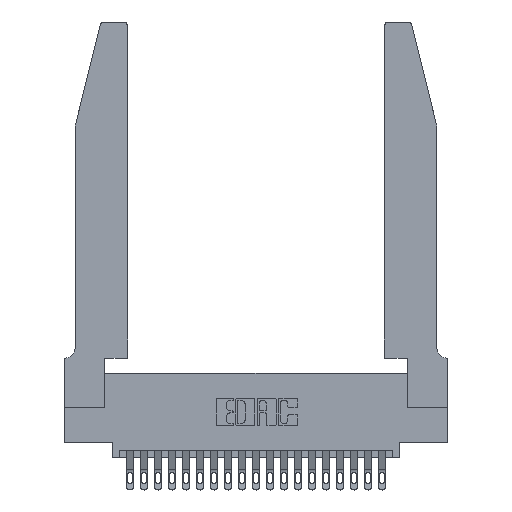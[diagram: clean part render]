
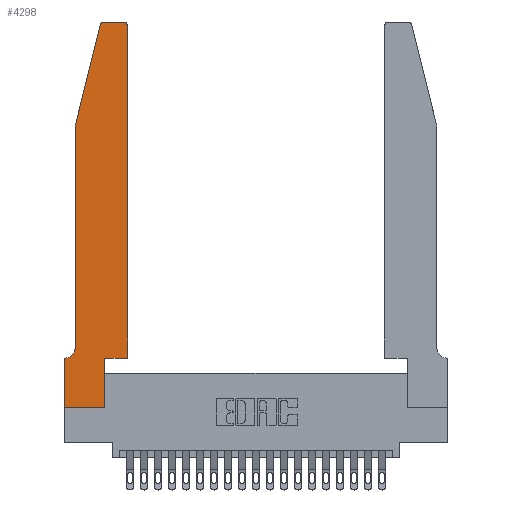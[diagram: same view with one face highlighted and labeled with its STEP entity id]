
A CAD part, top view. The second image highlights one B-rep face of the part: STEP entity #4298.
In plain terms, the highlighted planar face has unit normal (0, 0, 1).
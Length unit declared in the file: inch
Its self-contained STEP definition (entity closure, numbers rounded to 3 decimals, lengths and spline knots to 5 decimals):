
#197 = CARTESIAN_POINT ( 'NONE',  ( 0.4505, 0.35, 0.37 ) ) ;
#592 = LINE ( 'NONE', #1288, #1196 ) ;
#927 = ORIENTED_EDGE ( 'NONE', *, *, #7101, .T. ) ;
#1135 = CARTESIAN_POINT ( 'NONE',  ( 0.284, 2.72, 0.37 ) ) ;
#1196 = VECTOR ( 'NONE', #13981, 39.37008 ) ;
#1288 = CARTESIAN_POINT ( 'NONE',  ( 0., 0., 0.37 ) ) ;
#1310 = CARTESIAN_POINT ( 'NONE',  ( 0.0755, 0.35, 0.37 ) ) ;
#1815 = CARTESIAN_POINT ( 'NONE',  ( 0.0755, 2., 0.37 ) ) ;
#2028 = ORIENTED_EDGE ( 'NONE', *, *, #4688, .T. ) ;
#2301 = CARTESIAN_POINT ( 'NONE',  ( 0.0055, 0.35, 0.37 ) ) ;
#2383 = VERTEX_POINT ( 'NONE', #2521 ) ;
#2405 = CARTESIAN_POINT ( 'NONE',  ( 0.4205, 2.75, 0.37 ) ) ;
#2417 = CARTESIAN_POINT ( 'NONE',  ( 0., 0., 0.37 ) ) ;
#2521 = CARTESIAN_POINT ( 'NONE',  ( 0.2865, 0., 0.37 ) ) ;
#2837 = VECTOR ( 'NONE', #15884, 39.37008 ) ;
#2882 = CARTESIAN_POINT ( 'NONE',  ( 0.4505, 2.72, 0.37 ) ) ;
#3069 = DIRECTION ( 'NONE',  ( 1., 0., 0. ) ) ;
#3370 = CARTESIAN_POINT ( 'NONE',  ( 0.2865, 0.35, 0.37 ) ) ;
#3438 = AXIS2_PLACEMENT_3D ( 'NONE', #1135, #13840, #3069 ) ;
#3689 = LINE ( 'NONE', #4161, #21485 ) ;
#3809 = EDGE_CURVE ( 'NONE', #19338, #20474, #19629, .T. ) ;
#3865 = EDGE_CURVE ( 'NONE', #7633, #21622, #13322, .T. ) ;
#3909 = CIRCLE ( 'NONE', #22521, 0.07 ) ;
#4161 = CARTESIAN_POINT ( 'NONE',  ( 0.0755, 2., 0.37 ) ) ;
#4251 = CARTESIAN_POINT ( 'NONE',  ( 0.4505, 0.35, 0.37 ) ) ;
#4298 = ADVANCED_FACE ( 'NONE', ( #18496 ), #5028, .T. ) ;
#4553 = CARTESIAN_POINT ( 'NONE',  ( 0.25487, 2.72718, 0.37 ) ) ;
#4688 = EDGE_CURVE ( 'NONE', #5306, #2383, #10775, .T. ) ;
#5028 = PLANE ( 'NONE',  #18600 ) ;
#5179 = DIRECTION ( 'NONE',  ( 1., 0., 0. ) ) ;
#5306 = VERTEX_POINT ( 'NONE', #2417 ) ;
#5663 = VERTEX_POINT ( 'NONE', #1815 ) ;
#5896 = CIRCLE ( 'NONE', #3438, 0.03 ) ;
#5980 = VECTOR ( 'NONE', #18687, 39.37008 ) ;
#6511 = LINE ( 'NONE', #18050, #14353 ) ;
#6623 = EDGE_CURVE ( 'NONE', #16900, #19875, #5896, .T. ) ;
#7101 = EDGE_CURVE ( 'NONE', #21622, #19338, #19602, .T. ) ;
#7196 = ORIENTED_EDGE ( 'NONE', *, *, #20351, .T. ) ;
#7402 = EDGE_CURVE ( 'NONE', #2383, #7633, #16578, .T. ) ;
#7443 = CARTESIAN_POINT ( 'NONE',  ( 0.4205, 2.72, 0.37 ) ) ;
#7539 = DIRECTION ( 'NONE',  ( 0., -1., 0. ) ) ;
#7633 = VERTEX_POINT ( 'NONE', #9455 ) ;
#7802 = DIRECTION ( 'NONE',  ( -0.239, -0.971, 0. ) ) ;
#8399 = AXIS2_PLACEMENT_3D ( 'NONE', #7443, #19821, #9263 ) ;
#8579 = VECTOR ( 'NONE', #9417, 39.37008 ) ;
#8784 = CARTESIAN_POINT ( 'NONE',  ( 0.0055, 0.42, 0.37 ) ) ;
#8888 = ORIENTED_EDGE ( 'NONE', *, *, #9689, .T. ) ;
#9250 = CARTESIAN_POINT ( 'NONE',  ( 0.284, 2.75, 0.37 ) ) ;
#9263 = DIRECTION ( 'NONE',  ( 1., 0., 0. ) ) ;
#9417 = DIRECTION ( 'NONE',  ( 1., 0., 0. ) ) ;
#9455 = CARTESIAN_POINT ( 'NONE',  ( 0.2865, 0.35, 0.37 ) ) ;
#9689 = EDGE_CURVE ( 'NONE', #15528, #9977, #3909, .T. ) ;
#9833 = CARTESIAN_POINT ( 'NONE',  ( 0., 0., 0.37 ) ) ;
#9977 = VERTEX_POINT ( 'NONE', #2301 ) ;
#10240 = DIRECTION ( 'NONE',  ( -1., 0., 0. ) ) ;
#10323 = CARTESIAN_POINT ( 'NONE',  ( 0.2605, 2.75, 0.37 ) ) ;
#10567 = DIRECTION ( 'NONE',  ( -1., 0., 0. ) ) ;
#10775 = LINE ( 'NONE', #9833, #5980 ) ;
#11124 = CARTESIAN_POINT ( 'NONE',  ( 0.4505, 0.35, 0.37 ) ) ;
#11277 = CARTESIAN_POINT ( 'NONE',  ( 0., 0.35, 0.37 ) ) ;
#11360 = ORIENTED_EDGE ( 'NONE', *, *, #3809, .T. ) ;
#12433 = VECTOR ( 'NONE', #14005, 39.37008 ) ;
#13296 = ORIENTED_EDGE ( 'NONE', *, *, #6623, .T. ) ;
#13322 = LINE ( 'NONE', #11124, #8579 ) ;
#13417 = VERTEX_POINT ( 'NONE', #11277 ) ;
#13560 = ORIENTED_EDGE ( 'NONE', *, *, #7402, .T. ) ;
#13840 = DIRECTION ( 'NONE',  ( 0., 0., 1. ) ) ;
#13887 = EDGE_LOOP ( 'NONE', ( #20983, #13296, #22912, #7196, #8888, #18808, #19940, #2028, #13560, #14665, #927, #11360 ) ) ;
#13928 = VECTOR ( 'NONE', #10240, 39.37008 ) ;
#13981 = DIRECTION ( 'NONE',  ( 0., -1., 0. ) ) ;
#14005 = DIRECTION ( 'NONE',  ( -1., 0., 0. ) ) ;
#14353 = VECTOR ( 'NONE', #7539, 39.37008 ) ;
#14665 = ORIENTED_EDGE ( 'NONE', *, *, #3865, .T. ) ;
#15064 = EDGE_CURVE ( 'NONE', #9977, #13417, #17656, .T. ) ;
#15528 = VERTEX_POINT ( 'NONE', #18852 ) ;
#15797 = EDGE_CURVE ( 'NONE', #19875, #5663, #3689, .T. ) ;
#15884 = DIRECTION ( 'NONE',  ( 0., 1., 0. ) ) ;
#15897 = DIRECTION ( 'NONE',  ( 0., 0., 1. ) ) ;
#16578 = LINE ( 'NONE', #3370, #2837 ) ;
#16900 = VERTEX_POINT ( 'NONE', #9250 ) ;
#17486 = CARTESIAN_POINT ( 'NONE',  ( 0., 0.35, 0.37 ) ) ;
#17656 = LINE ( 'NONE', #1310, #12433 ) ;
#17710 = EDGE_CURVE ( 'NONE', #13417, #5306, #592, .T. ) ;
#17935 = VECTOR ( 'NONE', #18548, 39.37008 ) ;
#18050 = CARTESIAN_POINT ( 'NONE',  ( 0.0755, 2., 0.37 ) ) ;
#18496 = FACE_OUTER_BOUND ( 'NONE', #13887, .T. ) ;
#18548 = DIRECTION ( 'NONE',  ( 0., 1., 0. ) ) ;
#18600 = AXIS2_PLACEMENT_3D ( 'NONE', #17486, #15897, #5179 ) ;
#18687 = DIRECTION ( 'NONE',  ( 1., 0., 0. ) ) ;
#18808 = ORIENTED_EDGE ( 'NONE', *, *, #15064, .T. ) ;
#18852 = CARTESIAN_POINT ( 'NONE',  ( 0.0755, 0.42, 0.37 ) ) ;
#19338 = VERTEX_POINT ( 'NONE', #2882 ) ;
#19431 = EDGE_CURVE ( 'NONE', #20474, #16900, #22702, .T. ) ;
#19602 = LINE ( 'NONE', #4251, #17935 ) ;
#19629 = CIRCLE ( 'NONE', #8399, 0.03 ) ;
#19821 = DIRECTION ( 'NONE',  ( 0., 0., 1. ) ) ;
#19875 = VERTEX_POINT ( 'NONE', #4553 ) ;
#19940 = ORIENTED_EDGE ( 'NONE', *, *, #17710, .T. ) ;
#20351 = EDGE_CURVE ( 'NONE', #5663, #15528, #6511, .T. ) ;
#20474 = VERTEX_POINT ( 'NONE', #2405 ) ;
#20983 = ORIENTED_EDGE ( 'NONE', *, *, #19431, .T. ) ;
#21130 = DIRECTION ( 'NONE',  ( 0., 0., -1. ) ) ;
#21485 = VECTOR ( 'NONE', #7802, 39.37008 ) ;
#21622 = VERTEX_POINT ( 'NONE', #197 ) ;
#22521 = AXIS2_PLACEMENT_3D ( 'NONE', #8784, #21130, #10567 ) ;
#22702 = LINE ( 'NONE', #10323, #13928 ) ;
#22912 = ORIENTED_EDGE ( 'NONE', *, *, #15797, .T. ) ;
